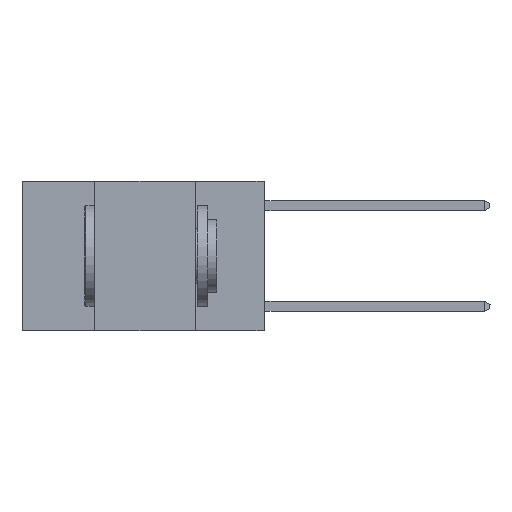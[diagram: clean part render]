
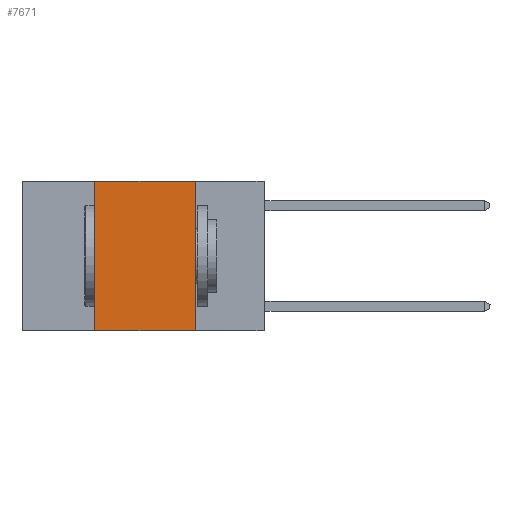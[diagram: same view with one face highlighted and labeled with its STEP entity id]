
A CAD part, left-side view. The second image highlights one B-rep face of the part: STEP entity #7671.
In plain terms, the highlighted planar face has unit normal (-1, 0, 0).
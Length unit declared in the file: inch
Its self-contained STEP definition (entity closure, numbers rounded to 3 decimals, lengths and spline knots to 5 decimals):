
#233 = VERTEX_POINT ( 'NONE', #9894 ) ;
#468 = ORIENTED_EDGE ( 'NONE', *, *, #6938, .F. ) ;
#1103 = VECTOR ( 'NONE', #13053, 39.37008 ) ;
#3563 = LINE ( 'NONE', #14570, #13830 ) ;
#3690 = CARTESIAN_POINT ( 'NONE',  ( 0., 0.17, -0.37 ) ) ;
#4132 = VERTEX_POINT ( 'NONE', #8720 ) ;
#4321 = DIRECTION ( 'NONE',  ( 0., 0., -1. ) ) ;
#4373 = ORIENTED_EDGE ( 'NONE', *, *, #5166, .F. ) ;
#5166 = EDGE_CURVE ( 'NONE', #4132, #233, #6913, .T. ) ;
#5246 = AXIS2_PLACEMENT_3D ( 'NONE', #17501, #8730, #4321 ) ;
#5425 = ORIENTED_EDGE ( 'NONE', *, *, #8640, .F. ) ;
#6913 = LINE ( 'NONE', #16850, #18514 ) ;
#6938 = EDGE_CURVE ( 'NONE', #233, #17394, #17098, .T. ) ;
#6969 = CARTESIAN_POINT ( 'NONE',  ( 0., 0.17, 0. ) ) ;
#7282 = DIRECTION ( 'NONE',  ( 0., -1., 0. ) ) ;
#7671 = ADVANCED_FACE ( 'NONE', ( #12468 ), #11627, .F. ) ;
#8218 = ORIENTED_EDGE ( 'NONE', *, *, #16945, .T. ) ;
#8326 = VECTOR ( 'NONE', #8391, 39.37008 ) ;
#8391 = DIRECTION ( 'NONE',  ( 0., 0., -1. ) ) ;
#8640 = EDGE_CURVE ( 'NONE', #17394, #10177, #12680, .T. ) ;
#8720 = CARTESIAN_POINT ( 'NONE',  ( 0., 0.42, -0.37 ) ) ;
#8730 = DIRECTION ( 'NONE',  ( 1., 0., 0. ) ) ;
#9894 = CARTESIAN_POINT ( 'NONE',  ( 0., 0.42, 0. ) ) ;
#10177 = VERTEX_POINT ( 'NONE', #3690 ) ;
#11585 = CARTESIAN_POINT ( 'NONE',  ( 0., 0.6, 0. ) ) ;
#11627 = PLANE ( 'NONE',  #5246 ) ;
#12397 = DIRECTION ( 'NONE',  ( 0., 0., 1. ) ) ;
#12468 = FACE_OUTER_BOUND ( 'NONE', #15784, .T. ) ;
#12680 = LINE ( 'NONE', #6969, #8326 ) ;
#13053 = DIRECTION ( 'NONE',  ( 0., -1., 0. ) ) ;
#13830 = VECTOR ( 'NONE', #7282, 39.37008 ) ;
#14570 = CARTESIAN_POINT ( 'NONE',  ( 0., 0.6, -0.37 ) ) ;
#15587 = CARTESIAN_POINT ( 'NONE',  ( 0., 0.17, 0. ) ) ;
#15784 = EDGE_LOOP ( 'NONE', ( #5425, #468, #4373, #8218 ) ) ;
#16850 = CARTESIAN_POINT ( 'NONE',  ( 0., 0.42, 0. ) ) ;
#16945 = EDGE_CURVE ( 'NONE', #4132, #10177, #3563, .T. ) ;
#17098 = LINE ( 'NONE', #11585, #1103 ) ;
#17394 = VERTEX_POINT ( 'NONE', #15587 ) ;
#17501 = CARTESIAN_POINT ( 'NONE',  ( 0., 0.6, 0. ) ) ;
#18514 = VECTOR ( 'NONE', #12397, 39.37008 ) ;
